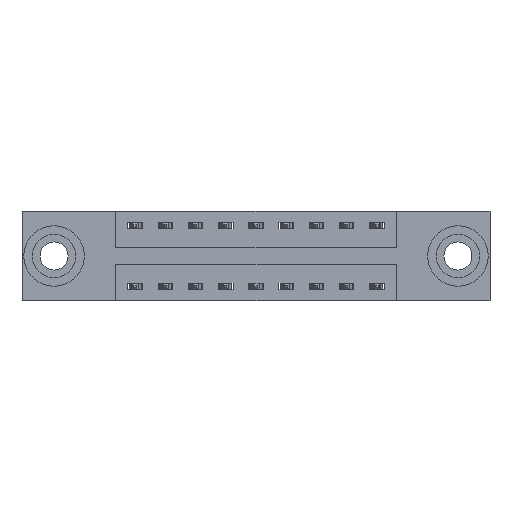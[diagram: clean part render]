
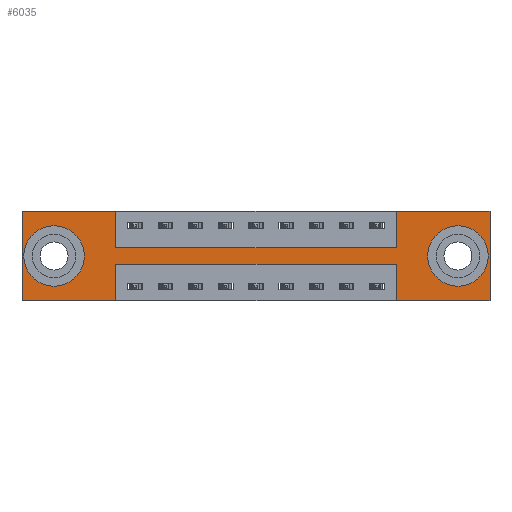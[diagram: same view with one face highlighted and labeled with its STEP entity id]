
A CAD part, front view. The second image highlights one B-rep face of the part: STEP entity #6035.
In plain terms, the highlighted planar face has unit normal (0, -1, 0).
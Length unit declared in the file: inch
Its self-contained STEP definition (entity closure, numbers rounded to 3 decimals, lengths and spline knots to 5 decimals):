
#8 = EDGE_CURVE ( 'NONE', #2205, #9681, #619, .T. ) ;
#52 = DIRECTION ( 'NONE',  ( 0., 1., 0. ) ) ;
#85 = ORIENTED_EDGE ( 'NONE', *, *, #8965, .F. ) ;
#321 = CARTESIAN_POINT ( 'NONE',  ( 1.5475, 0., -0.37 ) ) ;
#338 = ORIENTED_EDGE ( 'NONE', *, *, #368, .F. ) ;
#368 = EDGE_CURVE ( 'NONE', #6054, #8130, #6923, .T. ) ;
#383 = DIRECTION ( 'NONE',  ( 1., 0., 0. ) ) ;
#439 = DIRECTION ( 'NONE',  ( -1., 0., 0. ) ) ;
#544 = CIRCLE ( 'NONE', #4798, 0.078 ) ;
#619 = LINE ( 'NONE', #2393, #10859 ) ;
#621 = LINE ( 'NONE', #6954, #2975 ) ;
#915 = VECTOR ( 'NONE', #5707, 39.37008 ) ;
#1186 = VERTEX_POINT ( 'NONE', #9946 ) ;
#1212 = CIRCLE ( 'NONE', #7696, 0.078 ) ;
#1246 = CARTESIAN_POINT ( 'NONE',  ( 0.3875, 0., -0.15 ) ) ;
#1334 = EDGE_CURVE ( 'NONE', #9350, #4145, #3111, .T. ) ;
#1515 = VERTEX_POINT ( 'NONE', #5168 ) ;
#1518 = CARTESIAN_POINT ( 'NONE',  ( 1.5475, 0., 0. ) ) ;
#1556 = EDGE_CURVE ( 'NONE', #9805, #8012, #544, .T. ) ;
#1586 = DIRECTION ( 'NONE',  ( 0., 0., 1. ) ) ;
#1800 = DIRECTION ( 'NONE',  ( 0., 0., -1. ) ) ;
#2097 = LINE ( 'NONE', #1246, #5628 ) ;
#2152 = CARTESIAN_POINT ( 'NONE',  ( 0.3875, 0., 0. ) ) ;
#2205 = VERTEX_POINT ( 'NONE', #321 ) ;
#2338 = VERTEX_POINT ( 'NONE', #4202 ) ;
#2340 = CARTESIAN_POINT ( 'NONE',  ( 0.3875, 0., -0.37 ) ) ;
#2393 = CARTESIAN_POINT ( 'NONE',  ( 1.5475, 0., -0.37 ) ) ;
#2512 = CARTESIAN_POINT ( 'NONE',  ( 1.8025, 0., -0.185 ) ) ;
#2575 = ORIENTED_EDGE ( 'NONE', *, *, #4535, .F. ) ;
#2729 = VERTEX_POINT ( 'NONE', #3308 ) ;
#2733 = CARTESIAN_POINT ( 'NONE',  ( 0., 0., -0.37 ) ) ;
#2925 = DIRECTION ( 'NONE',  ( 0., 1., 0. ) ) ;
#2975 = VECTOR ( 'NONE', #3167, 39.37008 ) ;
#3074 = CARTESIAN_POINT ( 'NONE',  ( 1.8025, 0., -0.107 ) ) ;
#3111 = LINE ( 'NONE', #4817, #915 ) ;
#3167 = DIRECTION ( 'NONE',  ( 0., 0., -1. ) ) ;
#3214 = CARTESIAN_POINT ( 'NONE',  ( 0., 0., -0.37 ) ) ;
#3215 = CARTESIAN_POINT ( 'NONE',  ( 0., 0., 0. ) ) ;
#3234 = EDGE_LOOP ( 'NONE', ( #9530, #8186 ) ) ;
#3308 = CARTESIAN_POINT ( 'NONE',  ( 0.1325, 0., -0.107 ) ) ;
#3358 = VECTOR ( 'NONE', #3874, 39.37008 ) ;
#3493 = CARTESIAN_POINT ( 'NONE',  ( 0.3875, 0., -0.22 ) ) ;
#3533 = VECTOR ( 'NONE', #439, 39.37008 ) ;
#3826 = DIRECTION ( 'NONE',  ( 0., 0., 1. ) ) ;
#3874 = DIRECTION ( 'NONE',  ( -1., 0., 0. ) ) ;
#4016 = VECTOR ( 'NONE', #9502, 39.37008 ) ;
#4043 = PLANE ( 'NONE',  #5414 ) ;
#4145 = VERTEX_POINT ( 'NONE', #6591 ) ;
#4202 = CARTESIAN_POINT ( 'NONE',  ( 1.5475, 0., -0.15 ) ) ;
#4401 = DIRECTION ( 'NONE',  ( 0., 0., -1. ) ) ;
#4535 = EDGE_CURVE ( 'NONE', #10947, #10237, #6989, .T. ) ;
#4581 = EDGE_CURVE ( 'NONE', #9681, #6054, #6929, .T. ) ;
#4733 = ORIENTED_EDGE ( 'NONE', *, *, #6359, .F. ) ;
#4798 = AXIS2_PLACEMENT_3D ( 'NONE', #2512, #6098, #5348 ) ;
#4817 = CARTESIAN_POINT ( 'NONE',  ( 0.3875, 0., 0. ) ) ;
#4904 = AXIS2_PLACEMENT_3D ( 'NONE', #10217, #2925, #3826 ) ;
#4923 = CARTESIAN_POINT ( 'NONE',  ( 0., 0., 0. ) ) ;
#4956 = VECTOR ( 'NONE', #10297, 39.37008 ) ;
#4958 = VERTEX_POINT ( 'NONE', #6179 ) ;
#4972 = DIRECTION ( 'NONE',  ( 0., 1., 0. ) ) ;
#5106 = VERTEX_POINT ( 'NONE', #10963 ) ;
#5151 = CARTESIAN_POINT ( 'NONE',  ( 0.1325, 0., -0.185 ) ) ;
#5168 = CARTESIAN_POINT ( 'NONE',  ( 1.935, 0., -0.37 ) ) ;
#5348 = DIRECTION ( 'NONE',  ( 0., 0., -1. ) ) ;
#5414 = AXIS2_PLACEMENT_3D ( 'NONE', #3214, #10317, #10208 ) ;
#5554 = EDGE_CURVE ( 'NONE', #8130, #10947, #10091, .T. ) ;
#5569 = EDGE_CURVE ( 'NONE', #10237, #9350, #10035, .T. ) ;
#5628 = VECTOR ( 'NONE', #383, 39.37008 ) ;
#5707 = DIRECTION ( 'NONE',  ( 0., 0., -1. ) ) ;
#5835 = ORIENTED_EDGE ( 'NONE', *, *, #4581, .F. ) ;
#5857 = CARTESIAN_POINT ( 'NONE',  ( 0.3875, 0., -0.22 ) ) ;
#6018 = LINE ( 'NONE', #1518, #4016 ) ;
#6025 = FACE_BOUND ( 'NONE', #9854, .T. ) ;
#6035 = ADVANCED_FACE ( 'NONE', ( #10375, #6025, #6843 ), #4043, .T. ) ;
#6054 = VERTEX_POINT ( 'NONE', #5857 ) ;
#6058 = EDGE_CURVE ( 'NONE', #4958, #2729, #10158, .T. ) ;
#6098 = DIRECTION ( 'NONE',  ( 0., 1., 0. ) ) ;
#6179 = CARTESIAN_POINT ( 'NONE',  ( 0.1325, 0., -0.263 ) ) ;
#6359 = EDGE_CURVE ( 'NONE', #1515, #2205, #10718, .T. ) ;
#6391 = CARTESIAN_POINT ( 'NONE',  ( 1.5475, 0., -0.22 ) ) ;
#6591 = CARTESIAN_POINT ( 'NONE',  ( 0.3875, 0., -0.15 ) ) ;
#6789 = DIRECTION ( 'NONE',  ( 1., 0., 0. ) ) ;
#6843 = FACE_OUTER_BOUND ( 'NONE', #7276, .T. ) ;
#6848 = EDGE_CURVE ( 'NONE', #1186, #5106, #8651, .T. ) ;
#6923 = LINE ( 'NONE', #8790, #11419 ) ;
#6929 = LINE ( 'NONE', #3493, #8100 ) ;
#6954 = CARTESIAN_POINT ( 'NONE',  ( 1.935, 0., 0. ) ) ;
#6989 = LINE ( 'NONE', #11157, #4956 ) ;
#7068 = ORIENTED_EDGE ( 'NONE', *, *, #1334, .F. ) ;
#7263 = ORIENTED_EDGE ( 'NONE', *, *, #6058, .T. ) ;
#7276 = EDGE_LOOP ( 'NONE', ( #338, #5835, #9262, #4733, #85, #7292, #7323, #9564, #7068, #9794, #2575, #10493 ) ) ;
#7288 = ORIENTED_EDGE ( 'NONE', *, *, #10153, .T. ) ;
#7292 = ORIENTED_EDGE ( 'NONE', *, *, #6848, .F. ) ;
#7323 = ORIENTED_EDGE ( 'NONE', *, *, #7739, .F. ) ;
#7421 = CARTESIAN_POINT ( 'NONE',  ( 0., 0., -0.37 ) ) ;
#7647 = DIRECTION ( 'NONE',  ( 0., 0., 1. ) ) ;
#7681 = CIRCLE ( 'NONE', #4904, 0.078 ) ;
#7696 = AXIS2_PLACEMENT_3D ( 'NONE', #7820, #52, #4401 ) ;
#7739 = EDGE_CURVE ( 'NONE', #2338, #1186, #6018, .T. ) ;
#7820 = CARTESIAN_POINT ( 'NONE',  ( 1.8025, 0., -0.185 ) ) ;
#8012 = VERTEX_POINT ( 'NONE', #10613 ) ;
#8100 = VECTOR ( 'NONE', #10529, 39.37008 ) ;
#8130 = VERTEX_POINT ( 'NONE', #2340 ) ;
#8186 = ORIENTED_EDGE ( 'NONE', *, *, #8198, .T. ) ;
#8198 = EDGE_CURVE ( 'NONE', #8012, #9805, #1212, .T. ) ;
#8412 = CARTESIAN_POINT ( 'NONE',  ( 0., 0., -0.37 ) ) ;
#8651 = LINE ( 'NONE', #3215, #9822 ) ;
#8790 = CARTESIAN_POINT ( 'NONE',  ( 0.3875, 0., -0.37 ) ) ;
#8965 = EDGE_CURVE ( 'NONE', #5106, #1515, #621, .T. ) ;
#9228 = CARTESIAN_POINT ( 'NONE',  ( 0., 0., 0. ) ) ;
#9262 = ORIENTED_EDGE ( 'NONE', *, *, #8, .F. ) ;
#9330 = EDGE_CURVE ( 'NONE', #4145, #2338, #2097, .T. ) ;
#9350 = VERTEX_POINT ( 'NONE', #2152 ) ;
#9502 = DIRECTION ( 'NONE',  ( 0., 0., 1. ) ) ;
#9530 = ORIENTED_EDGE ( 'NONE', *, *, #1556, .T. ) ;
#9564 = ORIENTED_EDGE ( 'NONE', *, *, #9330, .F. ) ;
#9681 = VERTEX_POINT ( 'NONE', #6391 ) ;
#9794 = ORIENTED_EDGE ( 'NONE', *, *, #5569, .F. ) ;
#9805 = VERTEX_POINT ( 'NONE', #3074 ) ;
#9822 = VECTOR ( 'NONE', #6789, 39.37008 ) ;
#9854 = EDGE_LOOP ( 'NONE', ( #7288, #7263 ) ) ;
#9946 = CARTESIAN_POINT ( 'NONE',  ( 1.5475, 0., 0. ) ) ;
#10035 = LINE ( 'NONE', #9228, #10913 ) ;
#10091 = LINE ( 'NONE', #7421, #3358 ) ;
#10153 = EDGE_CURVE ( 'NONE', #2729, #4958, #7681, .T. ) ;
#10158 = CIRCLE ( 'NONE', #10709, 0.078 ) ;
#10208 = DIRECTION ( 'NONE',  ( 0., 0., -1. ) ) ;
#10217 = CARTESIAN_POINT ( 'NONE',  ( 0.1325, 0., -0.185 ) ) ;
#10237 = VERTEX_POINT ( 'NONE', #4923 ) ;
#10297 = DIRECTION ( 'NONE',  ( 0., 0., 1. ) ) ;
#10317 = DIRECTION ( 'NONE',  ( 0., -1., 0. ) ) ;
#10375 = FACE_BOUND ( 'NONE', #3234, .T. ) ;
#10493 = ORIENTED_EDGE ( 'NONE', *, *, #5554, .F. ) ;
#10529 = DIRECTION ( 'NONE',  ( -1., 0., 0. ) ) ;
#10613 = CARTESIAN_POINT ( 'NONE',  ( 1.8025, 0., -0.263 ) ) ;
#10709 = AXIS2_PLACEMENT_3D ( 'NONE', #5151, #4972, #1586 ) ;
#10718 = LINE ( 'NONE', #8412, #3533 ) ;
#10832 = DIRECTION ( 'NONE',  ( 1., 0., 0. ) ) ;
#10859 = VECTOR ( 'NONE', #7647, 39.37008 ) ;
#10913 = VECTOR ( 'NONE', #10832, 39.37008 ) ;
#10947 = VERTEX_POINT ( 'NONE', #2733 ) ;
#10963 = CARTESIAN_POINT ( 'NONE',  ( 1.935, 0., 0. ) ) ;
#11157 = CARTESIAN_POINT ( 'NONE',  ( 0., 0., 0. ) ) ;
#11419 = VECTOR ( 'NONE', #1800, 39.37008 ) ;
